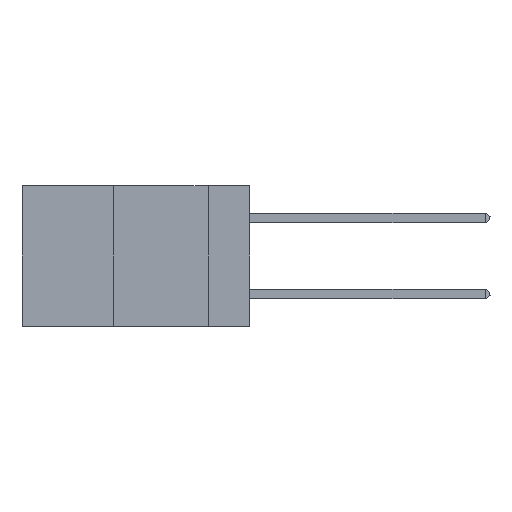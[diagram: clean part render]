
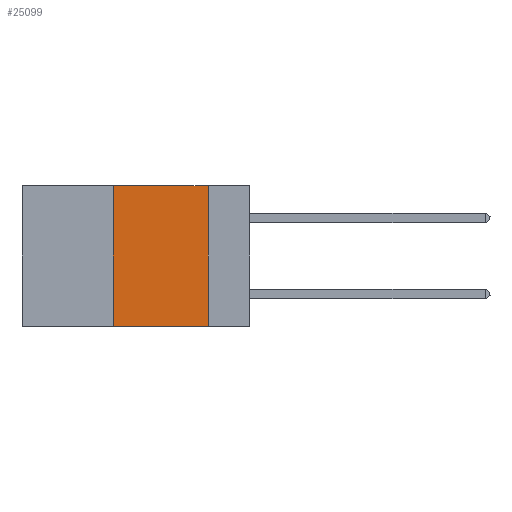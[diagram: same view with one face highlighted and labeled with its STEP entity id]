
A CAD part, left-side view. The second image highlights one B-rep face of the part: STEP entity #25099.
In plain terms, the highlighted planar face has unit normal (-1, 0, 0).
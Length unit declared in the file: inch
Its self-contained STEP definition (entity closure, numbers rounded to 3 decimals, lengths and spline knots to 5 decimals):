
#634 = DIRECTION ( 'NONE',  ( 0., 0., 1. ) ) ;
#802 = CARTESIAN_POINT ( 'NONE',  ( 0., 0.11, -0.37 ) ) ;
#1021 = VERTEX_POINT ( 'NONE', #802 ) ;
#1203 = EDGE_CURVE ( 'NONE', #24085, #1021, #1232, .T. ) ;
#1232 = LINE ( 'NONE', #14100, #14708 ) ;
#2206 = DIRECTION ( 'NONE',  ( 0., -1., 0. ) ) ;
#2592 = VECTOR ( 'NONE', #2206, 39.37008 ) ;
#4379 = CARTESIAN_POINT ( 'NONE',  ( 0., 0.6, 0. ) ) ;
#5676 = CARTESIAN_POINT ( 'NONE',  ( 0., 0.36, 0. ) ) ;
#6781 = LINE ( 'NONE', #5676, #15679 ) ;
#7239 = LINE ( 'NONE', #23930, #18970 ) ;
#7897 = VERTEX_POINT ( 'NONE', #31637 ) ;
#8650 = EDGE_CURVE ( 'NONE', #22623, #1021, #7239, .T. ) ;
#13281 = AXIS2_PLACEMENT_3D ( 'NONE', #4379, #14497, #31753 ) ;
#14074 = DIRECTION ( 'NONE',  ( 0., 0., -1. ) ) ;
#14100 = CARTESIAN_POINT ( 'NONE',  ( 0., 0.6, -0.37 ) ) ;
#14316 = EDGE_CURVE ( 'NONE', #7897, #22623, #16006, .T. ) ;
#14497 = DIRECTION ( 'NONE',  ( 1., 0., 0. ) ) ;
#14525 = EDGE_LOOP ( 'NONE', ( #20583, #21374, #22924, #17121 ) ) ;
#14708 = VECTOR ( 'NONE', #28882, 39.37008 ) ;
#15679 = VECTOR ( 'NONE', #634, 39.37008 ) ;
#16006 = LINE ( 'NONE', #32075, #2592 ) ;
#17054 = EDGE_CURVE ( 'NONE', #24085, #7897, #6781, .T. ) ;
#17121 = ORIENTED_EDGE ( 'NONE', *, *, #1203, .T. ) ;
#18970 = VECTOR ( 'NONE', #14074, 39.37008 ) ;
#20583 = ORIENTED_EDGE ( 'NONE', *, *, #8650, .F. ) ;
#21374 = ORIENTED_EDGE ( 'NONE', *, *, #14316, .F. ) ;
#21867 = PLANE ( 'NONE',  #13281 ) ;
#22475 = CARTESIAN_POINT ( 'NONE',  ( 0., 0.11, 0. ) ) ;
#22623 = VERTEX_POINT ( 'NONE', #22475 ) ;
#22924 = ORIENTED_EDGE ( 'NONE', *, *, #17054, .F. ) ;
#23930 = CARTESIAN_POINT ( 'NONE',  ( 0., 0.11, 0. ) ) ;
#24085 = VERTEX_POINT ( 'NONE', #30071 ) ;
#25099 = ADVANCED_FACE ( 'NONE', ( #25436 ), #21867, .F. ) ;
#25436 = FACE_OUTER_BOUND ( 'NONE', #14525, .T. ) ;
#28882 = DIRECTION ( 'NONE',  ( 0., -1., 0. ) ) ;
#30071 = CARTESIAN_POINT ( 'NONE',  ( 0., 0.36, -0.37 ) ) ;
#31637 = CARTESIAN_POINT ( 'NONE',  ( 0., 0.36, 0. ) ) ;
#31753 = DIRECTION ( 'NONE',  ( 0., 0., -1. ) ) ;
#32075 = CARTESIAN_POINT ( 'NONE',  ( 0., 0.6, 0. ) ) ;
